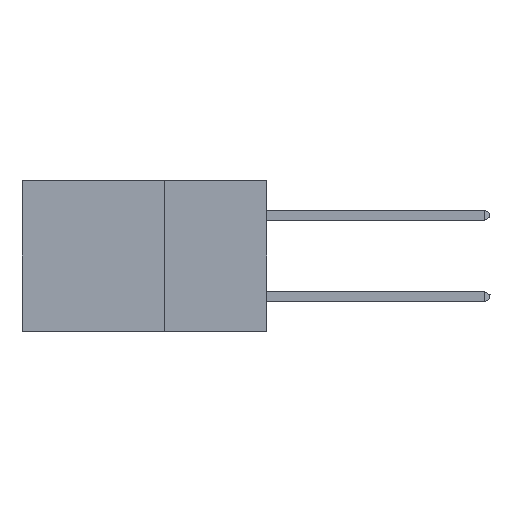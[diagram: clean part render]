
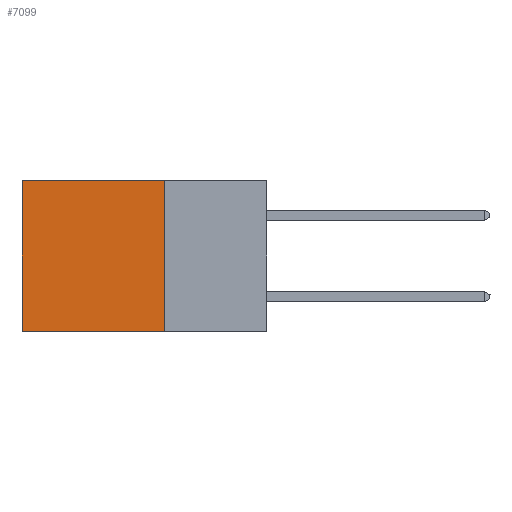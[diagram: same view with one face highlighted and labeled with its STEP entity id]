
A CAD part, left-side view. The second image highlights one B-rep face of the part: STEP entity #7099.
In plain terms, the highlighted planar face has unit normal (-1, 0, 0).
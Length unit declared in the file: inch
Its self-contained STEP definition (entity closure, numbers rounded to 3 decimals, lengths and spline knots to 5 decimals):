
#1525 = LINE ( 'NONE', #25978, #27337 ) ;
#1567 = VECTOR ( 'NONE', #16304, 39.37008 ) ;
#1927 = PLANE ( 'NONE',  #14436 ) ;
#2822 = ORIENTED_EDGE ( 'NONE', *, *, #21902, .T. ) ;
#2883 = LINE ( 'NONE', #19117, #1567 ) ;
#6283 = DIRECTION ( 'NONE',  ( 0., 1., 0. ) ) ;
#6401 = CARTESIAN_POINT ( 'NONE',  ( 0.2875, 0.25, 0. ) ) ;
#7099 = ADVANCED_FACE ( 'NONE', ( #29210 ), #1927, .F. ) ;
#8497 = VERTEX_POINT ( 'NONE', #20355 ) ;
#9944 = EDGE_CURVE ( 'NONE', #12316, #23322, #2883, .T. ) ;
#10158 = CARTESIAN_POINT ( 'NONE',  ( 0.2875, 0.25, 0. ) ) ;
#11594 = EDGE_CURVE ( 'NONE', #32128, #12316, #33404, .T. ) ;
#12316 = VERTEX_POINT ( 'NONE', #21950 ) ;
#14286 = VECTOR ( 'NONE', #24800, 39.37008 ) ;
#14436 = AXIS2_PLACEMENT_3D ( 'NONE', #10158, #18805, #24337 ) ;
#15983 = EDGE_CURVE ( 'NONE', #8497, #23322, #21727, .T. ) ;
#16304 = DIRECTION ( 'NONE',  ( 0., 1., 0. ) ) ;
#18805 = DIRECTION ( 'NONE',  ( 1., 0., 0. ) ) ;
#19117 = CARTESIAN_POINT ( 'NONE',  ( 0.2875, 0.25, -0.37 ) ) ;
#20355 = CARTESIAN_POINT ( 'NONE',  ( 0.2875, 0.6, 0. ) ) ;
#21372 = ORIENTED_EDGE ( 'NONE', *, *, #11594, .F. ) ;
#21727 = LINE ( 'NONE', #33369, #14286 ) ;
#21902 = EDGE_CURVE ( 'NONE', #32128, #8497, #1525, .T. ) ;
#21950 = CARTESIAN_POINT ( 'NONE',  ( 0.2875, 0.25, -0.37 ) ) ;
#23322 = VERTEX_POINT ( 'NONE', #34367 ) ;
#24337 = DIRECTION ( 'NONE',  ( 0., 0., -1. ) ) ;
#24800 = DIRECTION ( 'NONE',  ( 0., 0., -1. ) ) ;
#25938 = VECTOR ( 'NONE', #29277, 39.37008 ) ;
#25978 = CARTESIAN_POINT ( 'NONE',  ( 0.2875, 0.25, 0. ) ) ;
#27337 = VECTOR ( 'NONE', #6283, 39.37008 ) ;
#29210 = FACE_OUTER_BOUND ( 'NONE', #29720, .T. ) ;
#29277 = DIRECTION ( 'NONE',  ( 0., 0., -1. ) ) ;
#29720 = EDGE_LOOP ( 'NONE', ( #35849, #34856, #21372, #2822 ) ) ;
#32128 = VERTEX_POINT ( 'NONE', #33139 ) ;
#33139 = CARTESIAN_POINT ( 'NONE',  ( 0.2875, 0.25, 0. ) ) ;
#33369 = CARTESIAN_POINT ( 'NONE',  ( 0.2875, 0.6, 0. ) ) ;
#33404 = LINE ( 'NONE', #6401, #25938 ) ;
#34367 = CARTESIAN_POINT ( 'NONE',  ( 0.2875, 0.6, -0.37 ) ) ;
#34856 = ORIENTED_EDGE ( 'NONE', *, *, #9944, .F. ) ;
#35849 = ORIENTED_EDGE ( 'NONE', *, *, #15983, .T. ) ;
